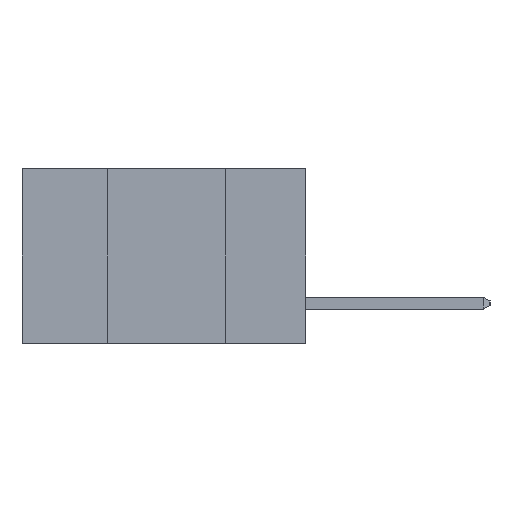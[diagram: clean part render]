
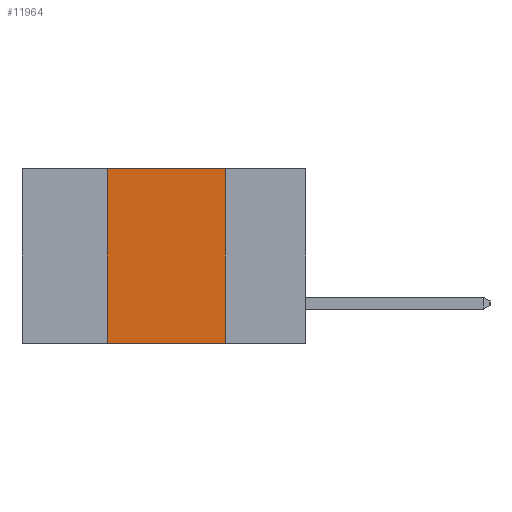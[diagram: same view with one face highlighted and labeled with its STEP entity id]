
A CAD part, left-side view. The second image highlights one B-rep face of the part: STEP entity #11964.
In plain terms, the highlighted planar face has unit normal (-1, 0, 0).
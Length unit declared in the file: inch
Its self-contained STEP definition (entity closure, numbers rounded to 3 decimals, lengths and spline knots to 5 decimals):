
#732 = EDGE_CURVE ( 'NONE', #3266, #23877, #22158, .T. ) ;
#752 = VECTOR ( 'NONE', #12136, 39.37008 ) ;
#2583 = CARTESIAN_POINT ( 'NONE',  ( 0., 0.17, -0.37 ) ) ;
#3266 = VERTEX_POINT ( 'NONE', #4654 ) ;
#4654 = CARTESIAN_POINT ( 'NONE',  ( 0., 0.42, -0.37 ) ) ;
#4739 = DIRECTION ( 'NONE',  ( 0., -1., 0. ) ) ;
#4756 = EDGE_CURVE ( 'NONE', #25235, #16291, #23442, .T. ) ;
#5212 = LINE ( 'NONE', #18490, #25154 ) ;
#5723 = ORIENTED_EDGE ( 'NONE', *, *, #4756, .F. ) ;
#5749 = CARTESIAN_POINT ( 'NONE',  ( 0., 0.17, 0. ) ) ;
#6294 = PLANE ( 'NONE',  #23641 ) ;
#8380 = DIRECTION ( 'NONE',  ( 1., 0., 0. ) ) ;
#8452 = CARTESIAN_POINT ( 'NONE',  ( 0., 0.42, 0. ) ) ;
#8759 = ORIENTED_EDGE ( 'NONE', *, *, #12769, .F. ) ;
#9289 = EDGE_LOOP ( 'NONE', ( #5723, #8759, #11349, #11110 ) ) ;
#9831 = CARTESIAN_POINT ( 'NONE',  ( 0., 0.17, 0. ) ) ;
#10657 = EDGE_CURVE ( 'NONE', #3266, #16291, #16660, .T. ) ;
#11110 = ORIENTED_EDGE ( 'NONE', *, *, #10657, .T. ) ;
#11349 = ORIENTED_EDGE ( 'NONE', *, *, #732, .F. ) ;
#11789 = DIRECTION ( 'NONE',  ( 0., 0., -1. ) ) ;
#11964 = ADVANCED_FACE ( 'NONE', ( #14613 ), #6294, .F. ) ;
#12136 = DIRECTION ( 'NONE',  ( 0., 0., 1. ) ) ;
#12239 = CARTESIAN_POINT ( 'NONE',  ( 0., 0.6, -0.37 ) ) ;
#12769 = EDGE_CURVE ( 'NONE', #23877, #25235, #5212, .T. ) ;
#13714 = CARTESIAN_POINT ( 'NONE',  ( 0., 0.42, 0. ) ) ;
#14258 = DIRECTION ( 'NONE',  ( 0., -1., 0. ) ) ;
#14613 = FACE_OUTER_BOUND ( 'NONE', #9289, .T. ) ;
#16291 = VERTEX_POINT ( 'NONE', #2583 ) ;
#16660 = LINE ( 'NONE', #12239, #21029 ) ;
#18466 = VECTOR ( 'NONE', #11789, 39.37008 ) ;
#18490 = CARTESIAN_POINT ( 'NONE',  ( 0., 0.6, 0. ) ) ;
#19908 = CARTESIAN_POINT ( 'NONE',  ( 0., 0.6, 0. ) ) ;
#21029 = VECTOR ( 'NONE', #14258, 39.37008 ) ;
#21783 = DIRECTION ( 'NONE',  ( 0., 0., -1. ) ) ;
#22158 = LINE ( 'NONE', #8452, #752 ) ;
#23442 = LINE ( 'NONE', #5749, #18466 ) ;
#23641 = AXIS2_PLACEMENT_3D ( 'NONE', #19908, #8380, #21783 ) ;
#23877 = VERTEX_POINT ( 'NONE', #13714 ) ;
#25154 = VECTOR ( 'NONE', #4739, 39.37008 ) ;
#25235 = VERTEX_POINT ( 'NONE', #9831 ) ;
